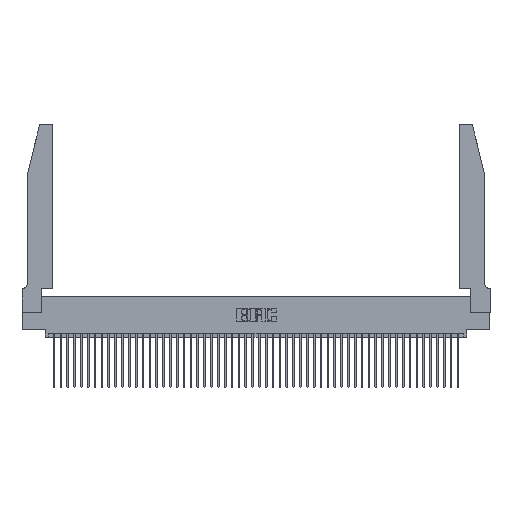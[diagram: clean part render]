
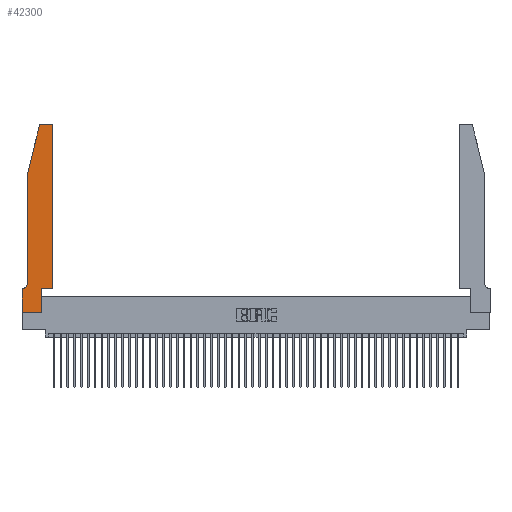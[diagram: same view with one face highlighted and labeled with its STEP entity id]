
A CAD part, top view. The second image highlights one B-rep face of the part: STEP entity #42300.
In plain terms, the highlighted planar face has unit normal (0, 0, 1).
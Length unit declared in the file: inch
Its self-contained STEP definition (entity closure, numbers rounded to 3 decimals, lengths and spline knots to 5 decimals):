
#631 = VECTOR ( 'NONE', #23216, 39.37008 ) ;
#852 = LINE ( 'NONE', #27841, #9940 ) ;
#1806 = ORIENTED_EDGE ( 'NONE', *, *, #18692, .T. ) ;
#2333 = CARTESIAN_POINT ( 'NONE',  ( 0.2865, 0.35, 0.37 ) ) ;
#2404 = CARTESIAN_POINT ( 'NONE',  ( 0.4205, 2.72, 0.37 ) ) ;
#2430 = VERTEX_POINT ( 'NONE', #12019 ) ;
#2655 = AXIS2_PLACEMENT_3D ( 'NONE', #38656, #15837, #42461 ) ;
#2803 = AXIS2_PLACEMENT_3D ( 'NONE', #2404, #29322, #6323 ) ;
#2842 = CARTESIAN_POINT ( 'NONE',  ( 0.0755, 0.42, 0.37 ) ) ;
#3506 = CIRCLE ( 'NONE', #2803, 0.03 ) ;
#4235 = ORIENTED_EDGE ( 'NONE', *, *, #25013, .T. ) ;
#5320 = VECTOR ( 'NONE', #16060, 39.37008 ) ;
#5849 = VERTEX_POINT ( 'NONE', #29216 ) ;
#6234 = DIRECTION ( 'NONE',  ( -0.239, -0.971, 0. ) ) ;
#6323 = DIRECTION ( 'NONE',  ( 1., 0., 0. ) ) ;
#6675 = ORIENTED_EDGE ( 'NONE', *, *, #26998, .T. ) ;
#7949 = CARTESIAN_POINT ( 'NONE',  ( 0.0755, 2., 0.37 ) ) ;
#8123 = VERTEX_POINT ( 'NONE', #2842 ) ;
#8207 = CARTESIAN_POINT ( 'NONE',  ( 0., 0., 0.37 ) ) ;
#9940 = VECTOR ( 'NONE', #24011, 39.37008 ) ;
#10007 = AXIS2_PLACEMENT_3D ( 'NONE', #42712, #19974, #46514 ) ;
#10784 = CARTESIAN_POINT ( 'NONE',  ( 0.284, 2.72, 0.37 ) ) ;
#10790 = ORIENTED_EDGE ( 'NONE', *, *, #41962, .T. ) ;
#10974 = VERTEX_POINT ( 'NONE', #13723 ) ;
#11269 = EDGE_CURVE ( 'NONE', #47633, #5849, #30104, .T. ) ;
#11955 = PLANE ( 'NONE',  #2655 ) ;
#12019 = CARTESIAN_POINT ( 'NONE',  ( 0.4205, 2.75, 0.37 ) ) ;
#12091 = LINE ( 'NONE', #13291, #41332 ) ;
#12172 = CARTESIAN_POINT ( 'NONE',  ( 0.2605, 2.75, 0.37 ) ) ;
#12173 = CARTESIAN_POINT ( 'NONE',  ( 0.4505, 0.35, 0.37 ) ) ;
#12263 = VECTOR ( 'NONE', #42681, 39.37008 ) ;
#12271 = EDGE_CURVE ( 'NONE', #17566, #10974, #18687, .T. ) ;
#13291 = CARTESIAN_POINT ( 'NONE',  ( 0.0755, 0.35, 0.37 ) ) ;
#13493 = VERTEX_POINT ( 'NONE', #7949 ) ;
#13723 = CARTESIAN_POINT ( 'NONE',  ( 0.2865, 0., 0.37 ) ) ;
#14348 = EDGE_CURVE ( 'NONE', #37944, #17566, #852, .T. ) ;
#14439 = ORIENTED_EDGE ( 'NONE', *, *, #12271, .T. ) ;
#14691 = DIRECTION ( 'NONE',  ( 1., 0., 0. ) ) ;
#15611 = LINE ( 'NONE', #12173, #5320 ) ;
#15837 = DIRECTION ( 'NONE',  ( 0., 0., 1. ) ) ;
#16060 = DIRECTION ( 'NONE',  ( 1., 0., 0. ) ) ;
#16082 = LINE ( 'NONE', #44486, #35156 ) ;
#17566 = VERTEX_POINT ( 'NONE', #8207 ) ;
#17748 = EDGE_CURVE ( 'NONE', #38141, #37944, #12091, .T. ) ;
#18427 = CIRCLE ( 'NONE', #10007, 0.07 ) ;
#18641 = ORIENTED_EDGE ( 'NONE', *, *, #45455, .T. ) ;
#18687 = LINE ( 'NONE', #31851, #37738 ) ;
#18692 = EDGE_CURVE ( 'NONE', #13493, #8123, #21046, .T. ) ;
#19409 = CARTESIAN_POINT ( 'NONE',  ( 0.4505, 0.35, 0.37 ) ) ;
#19974 = DIRECTION ( 'NONE',  ( 0., 0., -1. ) ) ;
#20620 = CARTESIAN_POINT ( 'NONE',  ( 0., 0.35, 0.37 ) ) ;
#21046 = LINE ( 'NONE', #29922, #38862 ) ;
#21782 = CARTESIAN_POINT ( 'NONE',  ( 0.0055, 0.35, 0.37 ) ) ;
#21826 = ORIENTED_EDGE ( 'NONE', *, *, #43733, .T. ) ;
#22882 = CARTESIAN_POINT ( 'NONE',  ( 0.25487, 2.72718, 0.37 ) ) ;
#23216 = DIRECTION ( 'NONE',  ( 0., 1., 0. ) ) ;
#24011 = DIRECTION ( 'NONE',  ( 0., -1., 0. ) ) ;
#24024 = VERTEX_POINT ( 'NONE', #42916 ) ;
#25013 = EDGE_CURVE ( 'NONE', #29968, #13493, #16082, .T. ) ;
#25206 = ORIENTED_EDGE ( 'NONE', *, *, #11269, .T. ) ;
#26998 = EDGE_CURVE ( 'NONE', #24024, #29968, #31492, .T. ) ;
#27841 = CARTESIAN_POINT ( 'NONE',  ( 0., 0., 0.37 ) ) ;
#29076 = CARTESIAN_POINT ( 'NONE',  ( 0.4505, 0.35, 0.37 ) ) ;
#29216 = CARTESIAN_POINT ( 'NONE',  ( 0.4505, 2.72, 0.37 ) ) ;
#29322 = DIRECTION ( 'NONE',  ( 0., 0., 1. ) ) ;
#29922 = CARTESIAN_POINT ( 'NONE',  ( 0.0755, 2., 0.37 ) ) ;
#29968 = VERTEX_POINT ( 'NONE', #22882 ) ;
#30104 = LINE ( 'NONE', #19409, #631 ) ;
#31492 = CIRCLE ( 'NONE', #41371, 0.03 ) ;
#31851 = CARTESIAN_POINT ( 'NONE',  ( 0., 0., 0.37 ) ) ;
#33048 = DIRECTION ( 'NONE',  ( 0., 1., 0. ) ) ;
#33735 = DIRECTION ( 'NONE',  ( 0., -1., 0. ) ) ;
#34153 = ORIENTED_EDGE ( 'NONE', *, *, #14348, .T. ) ;
#34237 = CARTESIAN_POINT ( 'NONE',  ( 0.2865, 0.35, 0.37 ) ) ;
#35156 = VECTOR ( 'NONE', #6234, 39.37008 ) ;
#35674 = DIRECTION ( 'NONE',  ( 1., 0., 0. ) ) ;
#35720 = EDGE_CURVE ( 'NONE', #5849, #2430, #3506, .T. ) ;
#36557 = ORIENTED_EDGE ( 'NONE', *, *, #17748, .T. ) ;
#37530 = DIRECTION ( 'NONE',  ( 0., 0., 1. ) ) ;
#37604 = EDGE_LOOP ( 'NONE', ( #21826, #6675, #4235, #1806, #40134, #36557, #34153, #14439, #10790, #18641, #25206, #47136 ) ) ;
#37738 = VECTOR ( 'NONE', #35674, 39.37008 ) ;
#37815 = EDGE_CURVE ( 'NONE', #8123, #38141, #18427, .T. ) ;
#37944 = VERTEX_POINT ( 'NONE', #20620 ) ;
#38107 = VECTOR ( 'NONE', #33048, 39.37008 ) ;
#38141 = VERTEX_POINT ( 'NONE', #21782 ) ;
#38656 = CARTESIAN_POINT ( 'NONE',  ( 0., 0.35, 0.37 ) ) ;
#38862 = VECTOR ( 'NONE', #33735, 39.37008 ) ;
#40134 = ORIENTED_EDGE ( 'NONE', *, *, #37815, .T. ) ;
#41210 = VERTEX_POINT ( 'NONE', #34237 ) ;
#41332 = VECTOR ( 'NONE', #47573, 39.37008 ) ;
#41371 = AXIS2_PLACEMENT_3D ( 'NONE', #10784, #37530, #14691 ) ;
#41493 = LINE ( 'NONE', #12172, #12263 ) ;
#41962 = EDGE_CURVE ( 'NONE', #10974, #41210, #48212, .T. ) ;
#42300 = ADVANCED_FACE ( 'NONE', ( #42824 ), #11955, .T. ) ;
#42461 = DIRECTION ( 'NONE',  ( 1., 0., 0. ) ) ;
#42681 = DIRECTION ( 'NONE',  ( -1., 0., 0. ) ) ;
#42712 = CARTESIAN_POINT ( 'NONE',  ( 0.0055, 0.42, 0.37 ) ) ;
#42824 = FACE_OUTER_BOUND ( 'NONE', #37604, .T. ) ;
#42916 = CARTESIAN_POINT ( 'NONE',  ( 0.284, 2.75, 0.37 ) ) ;
#43733 = EDGE_CURVE ( 'NONE', #2430, #24024, #41493, .T. ) ;
#44486 = CARTESIAN_POINT ( 'NONE',  ( 0.0755, 2., 0.37 ) ) ;
#45455 = EDGE_CURVE ( 'NONE', #41210, #47633, #15611, .T. ) ;
#46514 = DIRECTION ( 'NONE',  ( -1., 0., 0. ) ) ;
#47136 = ORIENTED_EDGE ( 'NONE', *, *, #35720, .T. ) ;
#47573 = DIRECTION ( 'NONE',  ( -1., 0., 0. ) ) ;
#47633 = VERTEX_POINT ( 'NONE', #29076 ) ;
#48212 = LINE ( 'NONE', #2333, #38107 ) ;
